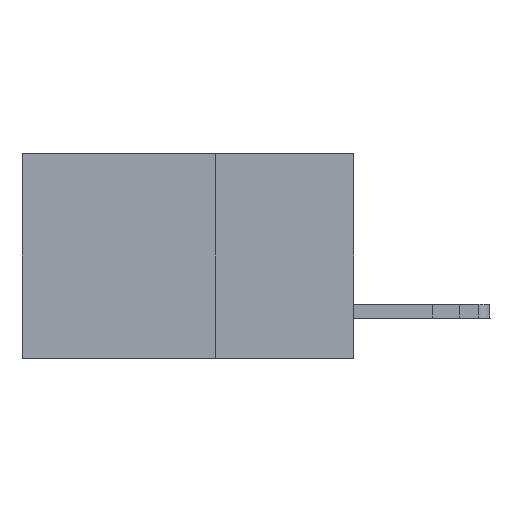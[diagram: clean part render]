
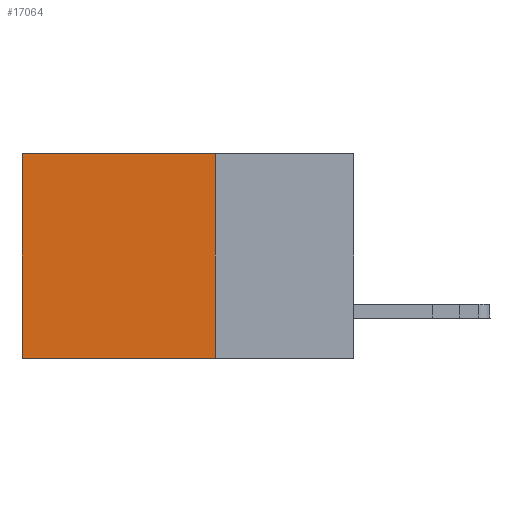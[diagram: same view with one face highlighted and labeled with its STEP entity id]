
A CAD part, left-side view. The second image highlights one B-rep face of the part: STEP entity #17064.
In plain terms, the highlighted planar face has unit normal (-1, 0, 0).
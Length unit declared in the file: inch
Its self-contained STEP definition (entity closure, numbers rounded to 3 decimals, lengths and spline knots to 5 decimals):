
#430 = LINE ( 'NONE', #7204, #7151 ) ;
#873 = CARTESIAN_POINT ( 'NONE',  ( 0.2875, 0.25, 0. ) ) ;
#1188 = LINE ( 'NONE', #3584, #16196 ) ;
#2685 = AXIS2_PLACEMENT_3D ( 'NONE', #20046, #6269, #6182 ) ;
#2880 = EDGE_LOOP ( 'NONE', ( #7963, #23001, #3297, #3196 ) ) ;
#3196 = ORIENTED_EDGE ( 'NONE', *, *, #3417, .T. ) ;
#3297 = ORIENTED_EDGE ( 'NONE', *, *, #16636, .F. ) ;
#3417 = EDGE_CURVE ( 'NONE', #5330, #7419, #1188, .T. ) ;
#3584 = CARTESIAN_POINT ( 'NONE',  ( 0.2875, 0.25, 0. ) ) ;
#5330 = VERTEX_POINT ( 'NONE', #18009 ) ;
#5349 = VERTEX_POINT ( 'NONE', #24470 ) ;
#5411 = LINE ( 'NONE', #14282, #20510 ) ;
#5605 = DIRECTION ( 'NONE',  ( 0., 1., 0. ) ) ;
#6182 = DIRECTION ( 'NONE',  ( 0., 0., -1. ) ) ;
#6269 = DIRECTION ( 'NONE',  ( 1., 0., 0. ) ) ;
#7048 = EDGE_CURVE ( 'NONE', #7419, #5349, #5411, .T. ) ;
#7151 = VECTOR ( 'NONE', #24694, 39.37008 ) ;
#7204 = CARTESIAN_POINT ( 'NONE',  ( 0.2875, 0.25, -0.37 ) ) ;
#7419 = VERTEX_POINT ( 'NONE', #18335 ) ;
#7963 = ORIENTED_EDGE ( 'NONE', *, *, #7048, .T. ) ;
#8162 = PLANE ( 'NONE',  #2685 ) ;
#8627 = DIRECTION ( 'NONE',  ( 0., 0., -1. ) ) ;
#8725 = VERTEX_POINT ( 'NONE', #9436 ) ;
#9436 = CARTESIAN_POINT ( 'NONE',  ( 0.2875, 0.25, -0.37 ) ) ;
#10247 = VECTOR ( 'NONE', #24547, 39.37008 ) ;
#13922 = LINE ( 'NONE', #873, #10247 ) ;
#14282 = CARTESIAN_POINT ( 'NONE',  ( 0.2875, 0.6, 0. ) ) ;
#16196 = VECTOR ( 'NONE', #5605, 39.37008 ) ;
#16636 = EDGE_CURVE ( 'NONE', #5330, #8725, #13922, .T. ) ;
#17064 = ADVANCED_FACE ( 'NONE', ( #21822 ), #8162, .F. ) ;
#18009 = CARTESIAN_POINT ( 'NONE',  ( 0.2875, 0.25, 0. ) ) ;
#18335 = CARTESIAN_POINT ( 'NONE',  ( 0.2875, 0.6, 0. ) ) ;
#20046 = CARTESIAN_POINT ( 'NONE',  ( 0.2875, 0.25, 0. ) ) ;
#20510 = VECTOR ( 'NONE', #8627, 39.37008 ) ;
#21822 = FACE_OUTER_BOUND ( 'NONE', #2880, .T. ) ;
#22691 = EDGE_CURVE ( 'NONE', #8725, #5349, #430, .T. ) ;
#23001 = ORIENTED_EDGE ( 'NONE', *, *, #22691, .F. ) ;
#24470 = CARTESIAN_POINT ( 'NONE',  ( 0.2875, 0.6, -0.37 ) ) ;
#24547 = DIRECTION ( 'NONE',  ( 0., 0., -1. ) ) ;
#24694 = DIRECTION ( 'NONE',  ( 0., 1., 0. ) ) ;
